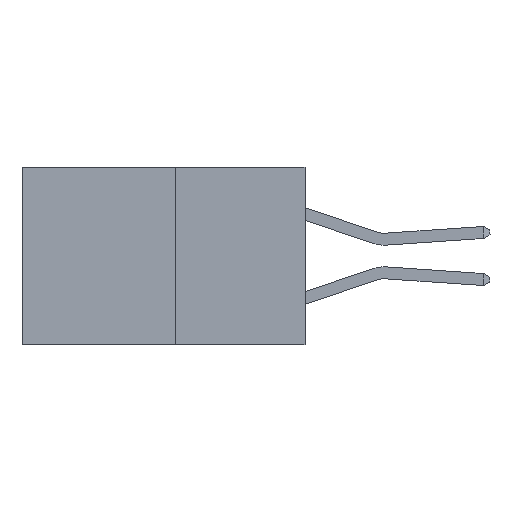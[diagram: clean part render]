
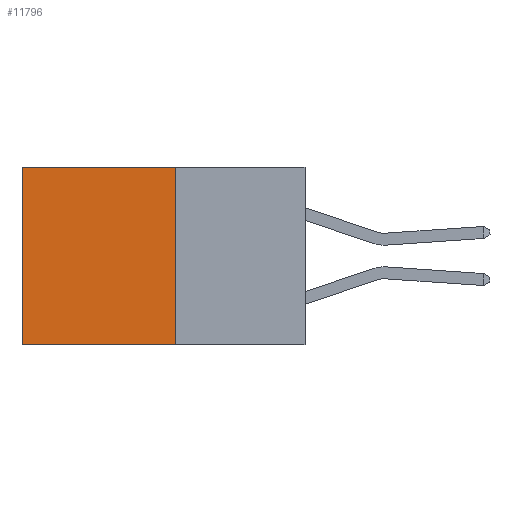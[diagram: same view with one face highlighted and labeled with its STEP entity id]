
A CAD part, left-side view. The second image highlights one B-rep face of the part: STEP entity #11796.
In plain terms, the highlighted planar face has unit normal (-1, 0, 0).
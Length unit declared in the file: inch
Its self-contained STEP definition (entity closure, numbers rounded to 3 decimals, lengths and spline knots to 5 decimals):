
#976 = EDGE_CURVE ( 'NONE', #5138, #11304, #18709, .T. ) ;
#1210 = ORIENTED_EDGE ( 'NONE', *, *, #976, .T. ) ;
#1579 = DIRECTION ( 'NONE',  ( 0., 0., -1. ) ) ;
#1748 = CARTESIAN_POINT ( 'NONE',  ( 0.277, 0.59, -0.37 ) ) ;
#3593 = CARTESIAN_POINT ( 'NONE',  ( 0.277, 0.27, 0. ) ) ;
#4824 = ORIENTED_EDGE ( 'NONE', *, *, #9846, .F. ) ;
#5138 = VERTEX_POINT ( 'NONE', #3593 ) ;
#5210 = EDGE_CURVE ( 'NONE', #11304, #26235, #10695, .T. ) ;
#6002 = VECTOR ( 'NONE', #15201, 39.37008 ) ;
#6431 = EDGE_CURVE ( 'NONE', #18542, #26235, #22712, .T. ) ;
#6838 = DIRECTION ( 'NONE',  ( 0., 0., -1. ) ) ;
#8704 = DIRECTION ( 'NONE',  ( 0., 1., 0. ) ) ;
#9140 = DIRECTION ( 'NONE',  ( 0., 0., -1. ) ) ;
#9846 = EDGE_CURVE ( 'NONE', #5138, #18542, #15655, .T. ) ;
#10695 = LINE ( 'NONE', #1748, #22640 ) ;
#11304 = VERTEX_POINT ( 'NONE', #26454 ) ;
#11796 = ADVANCED_FACE ( 'NONE', ( #28638 ), #28045, .F. ) ;
#13819 = CARTESIAN_POINT ( 'NONE',  ( 0.277, 0.27, -0.37 ) ) ;
#14929 = VECTOR ( 'NONE', #6838, 39.37008 ) ;
#15123 = CARTESIAN_POINT ( 'NONE',  ( 0.277, 0.59, -0.37 ) ) ;
#15201 = DIRECTION ( 'NONE',  ( 0., 1., 0. ) ) ;
#15655 = LINE ( 'NONE', #16309, #14929 ) ;
#16309 = CARTESIAN_POINT ( 'NONE',  ( 0.277, 0.27, -0.37 ) ) ;
#16371 = VECTOR ( 'NONE', #8704, 39.37008 ) ;
#16666 = AXIS2_PLACEMENT_3D ( 'NONE', #13819, #23407, #9140 ) ;
#18542 = VERTEX_POINT ( 'NONE', #26653 ) ;
#18709 = LINE ( 'NONE', #25674, #6002 ) ;
#19260 = ORIENTED_EDGE ( 'NONE', *, *, #5210, .T. ) ;
#21629 = EDGE_LOOP ( 'NONE', ( #19260, #24101, #4824, #1210 ) ) ;
#22640 = VECTOR ( 'NONE', #1579, 39.37008 ) ;
#22712 = LINE ( 'NONE', #27727, #16371 ) ;
#23407 = DIRECTION ( 'NONE',  ( 1., 0., 0. ) ) ;
#24101 = ORIENTED_EDGE ( 'NONE', *, *, #6431, .F. ) ;
#25674 = CARTESIAN_POINT ( 'NONE',  ( 0.277, 0.27, 0. ) ) ;
#26235 = VERTEX_POINT ( 'NONE', #15123 ) ;
#26454 = CARTESIAN_POINT ( 'NONE',  ( 0.277, 0.59, 0. ) ) ;
#26653 = CARTESIAN_POINT ( 'NONE',  ( 0.277, 0.27, -0.37 ) ) ;
#27727 = CARTESIAN_POINT ( 'NONE',  ( 0.277, 0.27, -0.37 ) ) ;
#28045 = PLANE ( 'NONE',  #16666 ) ;
#28638 = FACE_OUTER_BOUND ( 'NONE', #21629, .T. ) ;
